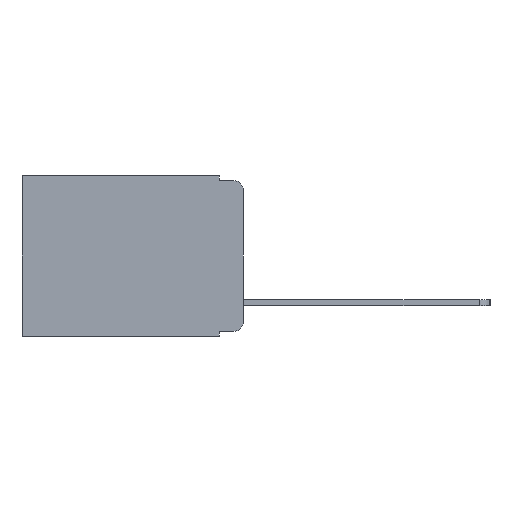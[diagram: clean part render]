
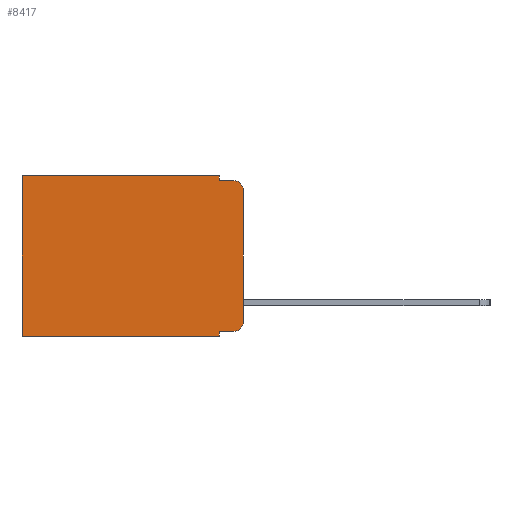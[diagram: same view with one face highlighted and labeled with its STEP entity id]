
A CAD part, left-side view. The second image highlights one B-rep face of the part: STEP entity #8417.
In plain terms, the highlighted planar face has unit normal (-1, 0, 0).
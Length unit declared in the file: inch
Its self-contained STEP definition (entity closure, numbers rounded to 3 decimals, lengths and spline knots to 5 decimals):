
#492 = LINE ( 'NONE', #9415, #11238 ) ;
#544 = CARTESIAN_POINT ( 'NONE',  ( 0.298, 0.02, -0.313 ) ) ;
#734 = LINE ( 'NONE', #12319, #8738 ) ;
#1158 = LINE ( 'NONE', #5632, #3605 ) ;
#1312 = ORIENTED_EDGE ( 'NONE', *, *, #2204, .F. ) ;
#1361 = LINE ( 'NONE', #5855, #11785 ) ;
#1468 = VECTOR ( 'NONE', #10498, 39.37008 ) ;
#1576 = DIRECTION ( 'NONE',  ( 0., 0., -1. ) ) ;
#1622 = ORIENTED_EDGE ( 'NONE', *, *, #4424, .T. ) ;
#1790 = VERTEX_POINT ( 'NONE', #13158 ) ;
#1944 = VECTOR ( 'NONE', #10575, 39.37008 ) ;
#2204 = EDGE_CURVE ( 'NONE', #3559, #9964, #1361, .T. ) ;
#2375 = CARTESIAN_POINT ( 'NONE',  ( 0.298, 0.473, 0. ) ) ;
#2406 = LINE ( 'NONE', #2375, #13132 ) ;
#2730 = CARTESIAN_POINT ( 'NONE',  ( 0.298, 0.02, -0.01 ) ) ;
#2759 = VERTEX_POINT ( 'NONE', #4089 ) ;
#2787 = CARTESIAN_POINT ( 'NONE',  ( 0.298, 0.051, -0.01 ) ) ;
#2990 = DIRECTION ( 'NONE',  ( -1., 0., 0. ) ) ;
#3178 = ORIENTED_EDGE ( 'NONE', *, *, #11483, .T. ) ;
#3556 = EDGE_CURVE ( 'NONE', #4722, #11936, #492, .T. ) ;
#3559 = VERTEX_POINT ( 'NONE', #10452 ) ;
#3605 = VECTOR ( 'NONE', #7736, 39.37008 ) ;
#3714 = EDGE_CURVE ( 'NONE', #2759, #6572, #4067, .T. ) ;
#3887 = DIRECTION ( 'NONE',  ( 0., 0., -1. ) ) ;
#4067 = LINE ( 'NONE', #11764, #10275 ) ;
#4089 = CARTESIAN_POINT ( 'NONE',  ( 0.298, 0., -0.03 ) ) ;
#4118 = ORIENTED_EDGE ( 'NONE', *, *, #4971, .T. ) ;
#4191 = DIRECTION ( 'NONE',  ( 0., 0., -1. ) ) ;
#4325 = CARTESIAN_POINT ( 'NONE',  ( 0.298, 0.051, -0.01 ) ) ;
#4424 = EDGE_CURVE ( 'NONE', #4906, #6572, #11539, .T. ) ;
#4482 = FACE_OUTER_BOUND ( 'NONE', #9503, .T. ) ;
#4722 = VERTEX_POINT ( 'NONE', #13399 ) ;
#4728 = LINE ( 'NONE', #4325, #1944 ) ;
#4906 = VERTEX_POINT ( 'NONE', #9602 ) ;
#4971 = EDGE_CURVE ( 'NONE', #11331, #9964, #2406, .T. ) ;
#5098 = ORIENTED_EDGE ( 'NONE', *, *, #12851, .F. ) ;
#5424 = EDGE_CURVE ( 'NONE', #1790, #3559, #7394, .T. ) ;
#5632 = CARTESIAN_POINT ( 'NONE',  ( 0.298, 0.051, -0.333 ) ) ;
#5855 = CARTESIAN_POINT ( 'NONE',  ( 0.298, 0., -0.343 ) ) ;
#6230 = ORIENTED_EDGE ( 'NONE', *, *, #12334, .T. ) ;
#6572 = VERTEX_POINT ( 'NONE', #8865 ) ;
#7000 = ORIENTED_EDGE ( 'NONE', *, *, #8501, .T. ) ;
#7025 = PLANE ( 'NONE',  #10723 ) ;
#7394 = LINE ( 'NONE', #10448, #1468 ) ;
#7421 = AXIS2_PLACEMENT_3D ( 'NONE', #544, #7881, #1576 ) ;
#7683 = DIRECTION ( 'NONE',  ( 0., 0., -1. ) ) ;
#7736 = DIRECTION ( 'NONE',  ( 0., -1., 0. ) ) ;
#7881 = DIRECTION ( 'NONE',  ( -1., 0., 0. ) ) ;
#7888 = VERTEX_POINT ( 'NONE', #2730 ) ;
#7943 = CARTESIAN_POINT ( 'NONE',  ( 0.298, 0.473, 0. ) ) ;
#8417 = ADVANCED_FACE ( 'NONE', ( #4482 ), #7025, .F. ) ;
#8501 = EDGE_CURVE ( 'NONE', #4722, #11331, #734, .T. ) ;
#8738 = VECTOR ( 'NONE', #13336, 39.37008 ) ;
#8865 = CARTESIAN_POINT ( 'NONE',  ( 0.298, 0., -0.313 ) ) ;
#8943 = DIRECTION ( 'NONE',  ( 0., 1., 0. ) ) ;
#9256 = CARTESIAN_POINT ( 'NONE',  ( 0.298, 0.02, -0.03 ) ) ;
#9415 = CARTESIAN_POINT ( 'NONE',  ( 0.298, 0.051, 0. ) ) ;
#9503 = EDGE_LOOP ( 'NONE', ( #11174, #3178, #5098, #12972, #7000, #4118, #1312, #9750, #6230, #1622 ) ) ;
#9602 = CARTESIAN_POINT ( 'NONE',  ( 0.298, 0.02, -0.333 ) ) ;
#9750 = ORIENTED_EDGE ( 'NONE', *, *, #5424, .F. ) ;
#9964 = VERTEX_POINT ( 'NONE', #12711 ) ;
#10126 = DIRECTION ( 'NONE',  ( 1., 0., 0. ) ) ;
#10275 = VECTOR ( 'NONE', #7683, 39.37008 ) ;
#10301 = DIRECTION ( 'NONE',  ( 0., 0., -1. ) ) ;
#10412 = AXIS2_PLACEMENT_3D ( 'NONE', #9256, #2990, #10301 ) ;
#10448 = CARTESIAN_POINT ( 'NONE',  ( 0.298, 0.051, 0. ) ) ;
#10452 = CARTESIAN_POINT ( 'NONE',  ( 0.298, 0.051, -0.343 ) ) ;
#10498 = DIRECTION ( 'NONE',  ( 0., 0., -1. ) ) ;
#10575 = DIRECTION ( 'NONE',  ( 0., -1., 0. ) ) ;
#10723 = AXIS2_PLACEMENT_3D ( 'NONE', #12155, #10126, #3887 ) ;
#11174 = ORIENTED_EDGE ( 'NONE', *, *, #3714, .F. ) ;
#11238 = VECTOR ( 'NONE', #4191, 39.37008 ) ;
#11331 = VERTEX_POINT ( 'NONE', #7943 ) ;
#11483 = EDGE_CURVE ( 'NONE', #2759, #7888, #11942, .T. ) ;
#11539 = CIRCLE ( 'NONE', #7421, 0.02 ) ;
#11764 = CARTESIAN_POINT ( 'NONE',  ( 0.298, 0., 0. ) ) ;
#11777 = DIRECTION ( 'NONE',  ( 0., 0., -1. ) ) ;
#11785 = VECTOR ( 'NONE', #8943, 39.37008 ) ;
#11936 = VERTEX_POINT ( 'NONE', #2787 ) ;
#11942 = CIRCLE ( 'NONE', #10412, 0.02 ) ;
#12155 = CARTESIAN_POINT ( 'NONE',  ( 0.298, 0., 0. ) ) ;
#12319 = CARTESIAN_POINT ( 'NONE',  ( 0.298, 0., 0. ) ) ;
#12334 = EDGE_CURVE ( 'NONE', #1790, #4906, #1158, .T. ) ;
#12711 = CARTESIAN_POINT ( 'NONE',  ( 0.298, 0.473, -0.343 ) ) ;
#12851 = EDGE_CURVE ( 'NONE', #11936, #7888, #4728, .T. ) ;
#12972 = ORIENTED_EDGE ( 'NONE', *, *, #3556, .F. ) ;
#13132 = VECTOR ( 'NONE', #11777, 39.37008 ) ;
#13158 = CARTESIAN_POINT ( 'NONE',  ( 0.298, 0.051, -0.333 ) ) ;
#13336 = DIRECTION ( 'NONE',  ( 0., 1., 0. ) ) ;
#13399 = CARTESIAN_POINT ( 'NONE',  ( 0.298, 0.051, 0. ) ) ;
